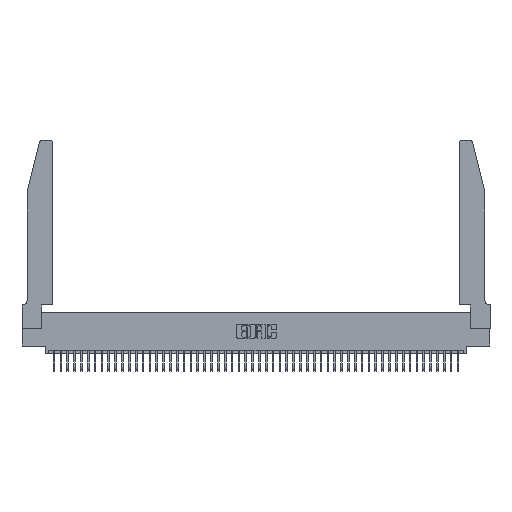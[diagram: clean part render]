
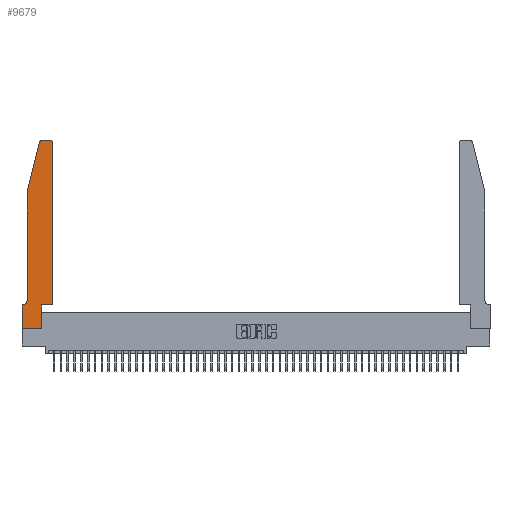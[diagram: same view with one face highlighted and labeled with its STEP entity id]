
A CAD part, top view. The second image highlights one B-rep face of the part: STEP entity #9679.
In plain terms, the highlighted planar face has unit normal (0, 0, 1).
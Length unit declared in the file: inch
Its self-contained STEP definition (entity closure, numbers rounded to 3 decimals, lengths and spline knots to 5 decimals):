
#1164 = ORIENTED_EDGE ( 'NONE', *, *, #11480, .T. ) ;
#1423 = VECTOR ( 'NONE', #49232, 39.37008 ) ;
#1550 = CARTESIAN_POINT ( 'NONE',  ( 0.0755, 2., 0.37 ) ) ;
#1667 = VERTEX_POINT ( 'NONE', #43333 ) ;
#1962 = CARTESIAN_POINT ( 'NONE',  ( 0.2865, 0.35, 0.37 ) ) ;
#2211 = EDGE_LOOP ( 'NONE', ( #12045, #18143, #49921, #26924, #1164, #15733, #34103, #9745, #26722, #32945, #42887, #28947 ) ) ;
#2620 = VERTEX_POINT ( 'NONE', #1550 ) ;
#2690 = LINE ( 'NONE', #9800, #1423 ) ;
#2851 = AXIS2_PLACEMENT_3D ( 'NONE', #8405, #32170, #8582 ) ;
#3363 = CARTESIAN_POINT ( 'NONE',  ( 0.284, 2.72, 0.37 ) ) ;
#3861 = EDGE_CURVE ( 'NONE', #41508, #18554, #28872, .T. ) ;
#4601 = CARTESIAN_POINT ( 'NONE',  ( 0.2865, 0.35, 0.37 ) ) ;
#4930 = CARTESIAN_POINT ( 'NONE',  ( 0.4505, 0.35, 0.37 ) ) ;
#5471 = DIRECTION ( 'NONE',  ( 0., 0., 1. ) ) ;
#5719 = EDGE_CURVE ( 'NONE', #41270, #41508, #24162, .T. ) ;
#7407 = DIRECTION ( 'NONE',  ( 1., 0., 0. ) ) ;
#8405 = CARTESIAN_POINT ( 'NONE',  ( 0., 0.35, 0.37 ) ) ;
#8582 = DIRECTION ( 'NONE',  ( 1., 0., 0. ) ) ;
#9679 = ADVANCED_FACE ( 'NONE', ( #42293 ), #12420, .T. ) ;
#9745 = ORIENTED_EDGE ( 'NONE', *, *, #18407, .T. ) ;
#9800 = CARTESIAN_POINT ( 'NONE',  ( 0., 0., 0.37 ) ) ;
#10731 = CARTESIAN_POINT ( 'NONE',  ( 0.284, 2.75, 0.37 ) ) ;
#11480 = EDGE_CURVE ( 'NONE', #1667, #29553, #35349, .T. ) ;
#12045 = ORIENTED_EDGE ( 'NONE', *, *, #15337, .T. ) ;
#12420 = PLANE ( 'NONE',  #2851 ) ;
#12470 = DIRECTION ( 'NONE',  ( 0., -1., 0. ) ) ;
#12513 = VERTEX_POINT ( 'NONE', #4601 ) ;
#13619 = VERTEX_POINT ( 'NONE', #37073 ) ;
#15251 = CARTESIAN_POINT ( 'NONE',  ( 0.4505, 0.35, 0.37 ) ) ;
#15337 = EDGE_CURVE ( 'NONE', #18554, #35060, #27570, .T. ) ;
#15733 = ORIENTED_EDGE ( 'NONE', *, *, #19765, .T. ) ;
#18143 = ORIENTED_EDGE ( 'NONE', *, *, #44243, .T. ) ;
#18407 = EDGE_CURVE ( 'NONE', #13619, #32610, #2690, .T. ) ;
#18554 = VERTEX_POINT ( 'NONE', #42332 ) ;
#19303 = VECTOR ( 'NONE', #37643, 39.37008 ) ;
#19765 = EDGE_CURVE ( 'NONE', #29553, #47128, #48889, .T. ) ;
#21118 = CARTESIAN_POINT ( 'NONE',  ( 0.0755, 2., 0.37 ) ) ;
#21207 = CARTESIAN_POINT ( 'NONE',  ( 0.4505, 0.35, 0.37 ) ) ;
#21708 = DIRECTION ( 'NONE',  ( 0., 0., -1. ) ) ;
#22316 = AXIS2_PLACEMENT_3D ( 'NONE', #29167, #5471, #33119 ) ;
#22413 = CARTESIAN_POINT ( 'NONE',  ( 0.0055, 0.35, 0.37 ) ) ;
#23363 = CARTESIAN_POINT ( 'NONE',  ( 0.0755, 2., 0.37 ) ) ;
#24162 = LINE ( 'NONE', #21207, #43872 ) ;
#24339 = CARTESIAN_POINT ( 'NONE',  ( 0.2605, 2.75, 0.37 ) ) ;
#24341 = CARTESIAN_POINT ( 'NONE',  ( 0., 0., 0.37 ) ) ;
#25082 = DIRECTION ( 'NONE',  ( 0., -1., 0. ) ) ;
#25165 = DIRECTION ( 'NONE',  ( 0., 1., 0. ) ) ;
#25181 = VECTOR ( 'NONE', #12470, 39.37008 ) ;
#26336 = VECTOR ( 'NONE', #28294, 39.37008 ) ;
#26425 = LINE ( 'NONE', #24341, #25181 ) ;
#26722 = ORIENTED_EDGE ( 'NONE', *, *, #48227, .T. ) ;
#26924 = ORIENTED_EDGE ( 'NONE', *, *, #38808, .T. ) ;
#27513 = LINE ( 'NONE', #21118, #36775 ) ;
#27554 = CARTESIAN_POINT ( 'NONE',  ( 0.0755, 0.35, 0.37 ) ) ;
#27565 = CARTESIAN_POINT ( 'NONE',  ( 0.25487, 2.72718, 0.37 ) ) ;
#27570 = LINE ( 'NONE', #24339, #26336 ) ;
#28294 = DIRECTION ( 'NONE',  ( -1., 0., 0. ) ) ;
#28872 = CIRCLE ( 'NONE', #22316, 0.03 ) ;
#28947 = ORIENTED_EDGE ( 'NONE', *, *, #3861, .T. ) ;
#29063 = VECTOR ( 'NONE', #39234, 39.37008 ) ;
#29167 = CARTESIAN_POINT ( 'NONE',  ( 0.4205, 2.72, 0.37 ) ) ;
#29553 = VERTEX_POINT ( 'NONE', #22413 ) ;
#29724 = VERTEX_POINT ( 'NONE', #27565 ) ;
#29778 = LINE ( 'NONE', #1962, #19303 ) ;
#31042 = DIRECTION ( 'NONE',  ( 0., 0., 1. ) ) ;
#32170 = DIRECTION ( 'NONE',  ( 0., 0., 1. ) ) ;
#32610 = VERTEX_POINT ( 'NONE', #46883 ) ;
#32945 = ORIENTED_EDGE ( 'NONE', *, *, #40962, .T. ) ;
#33119 = DIRECTION ( 'NONE',  ( 1., 0., 0. ) ) ;
#33946 = CARTESIAN_POINT ( 'NONE',  ( 0.4505, 2.72, 0.37 ) ) ;
#34103 = ORIENTED_EDGE ( 'NONE', *, *, #44454, .T. ) ;
#35060 = VERTEX_POINT ( 'NONE', #10731 ) ;
#35349 = CIRCLE ( 'NONE', #44668, 0.07 ) ;
#36307 = CIRCLE ( 'NONE', #48738, 0.03 ) ;
#36775 = VECTOR ( 'NONE', #25082, 39.37008 ) ;
#37073 = CARTESIAN_POINT ( 'NONE',  ( 0., 0., 0.37 ) ) ;
#37643 = DIRECTION ( 'NONE',  ( 0., 1., 0. ) ) ;
#38461 = VECTOR ( 'NONE', #43391, 39.37008 ) ;
#38808 = EDGE_CURVE ( 'NONE', #2620, #1667, #27513, .T. ) ;
#38840 = DIRECTION ( 'NONE',  ( 1., 0., 0. ) ) ;
#39234 = DIRECTION ( 'NONE',  ( -0.239, -0.971, 0. ) ) ;
#39293 = CARTESIAN_POINT ( 'NONE',  ( 0., 0.35, 0.37 ) ) ;
#39704 = VECTOR ( 'NONE', #38840, 39.37008 ) ;
#40962 = EDGE_CURVE ( 'NONE', #12513, #41270, #50154, .T. ) ;
#41270 = VERTEX_POINT ( 'NONE', #4930 ) ;
#41508 = VERTEX_POINT ( 'NONE', #33946 ) ;
#42293 = FACE_OUTER_BOUND ( 'NONE', #2211, .T. ) ;
#42332 = CARTESIAN_POINT ( 'NONE',  ( 0.4205, 2.75, 0.37 ) ) ;
#42361 = EDGE_CURVE ( 'NONE', #29724, #2620, #47944, .T. ) ;
#42887 = ORIENTED_EDGE ( 'NONE', *, *, #5719, .T. ) ;
#43333 = CARTESIAN_POINT ( 'NONE',  ( 0.0755, 0.42, 0.37 ) ) ;
#43391 = DIRECTION ( 'NONE',  ( -1., 0., 0. ) ) ;
#43872 = VECTOR ( 'NONE', #25165, 39.37008 ) ;
#44243 = EDGE_CURVE ( 'NONE', #35060, #29724, #36307, .T. ) ;
#44454 = EDGE_CURVE ( 'NONE', #47128, #13619, #26425, .T. ) ;
#44668 = AXIS2_PLACEMENT_3D ( 'NONE', #45299, #21708, #49250 ) ;
#45299 = CARTESIAN_POINT ( 'NONE',  ( 0.0055, 0.42, 0.37 ) ) ;
#46883 = CARTESIAN_POINT ( 'NONE',  ( 0.2865, 0., 0.37 ) ) ;
#47128 = VERTEX_POINT ( 'NONE', #39293 ) ;
#47944 = LINE ( 'NONE', #23363, #29063 ) ;
#48227 = EDGE_CURVE ( 'NONE', #32610, #12513, #29778, .T. ) ;
#48738 = AXIS2_PLACEMENT_3D ( 'NONE', #3363, #31042, #7407 ) ;
#48889 = LINE ( 'NONE', #27554, #38461 ) ;
#49232 = DIRECTION ( 'NONE',  ( 1., 0., 0. ) ) ;
#49250 = DIRECTION ( 'NONE',  ( -1., 0., 0. ) ) ;
#49921 = ORIENTED_EDGE ( 'NONE', *, *, #42361, .T. ) ;
#50154 = LINE ( 'NONE', #15251, #39704 ) ;
